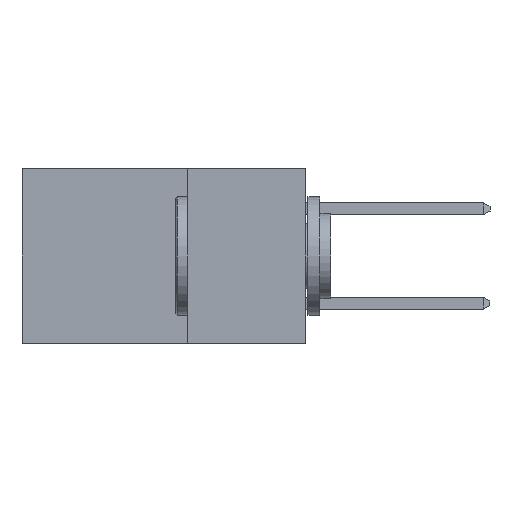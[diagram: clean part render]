
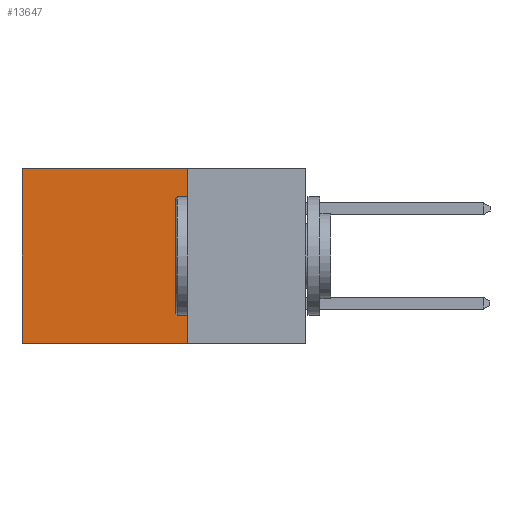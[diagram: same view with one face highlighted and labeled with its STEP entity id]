
A CAD part, left-side view. The second image highlights one B-rep face of the part: STEP entity #13647.
In plain terms, the highlighted planar face has unit normal (-1, 0, 0).
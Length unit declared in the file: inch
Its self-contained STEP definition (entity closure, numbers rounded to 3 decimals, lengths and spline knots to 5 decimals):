
#135 = EDGE_LOOP ( 'NONE', ( #23968, #1045, #19293, #12222 ) ) ;
#969 = CARTESIAN_POINT ( 'NONE',  ( 0.298, 0.25, -0.37 ) ) ;
#1045 = ORIENTED_EDGE ( 'NONE', *, *, #22893, .F. ) ;
#1444 = LINE ( 'NONE', #969, #5917 ) ;
#2767 = CARTESIAN_POINT ( 'NONE',  ( 0.298, 0.25, 0. ) ) ;
#2989 = CARTESIAN_POINT ( 'NONE',  ( 0.298, 0.25, 0. ) ) ;
#3025 = CARTESIAN_POINT ( 'NONE',  ( 0.298, 0.6, -0.37 ) ) ;
#3817 = EDGE_CURVE ( 'NONE', #9918, #7868, #16324, .T. ) ;
#3919 = VERTEX_POINT ( 'NONE', #2767 ) ;
#4996 = CARTESIAN_POINT ( 'NONE',  ( 0.298, 0.25, 0. ) ) ;
#5917 = VECTOR ( 'NONE', #16052, 39.37008 ) ;
#5967 = FACE_OUTER_BOUND ( 'NONE', #135, .T. ) ;
#6118 = AXIS2_PLACEMENT_3D ( 'NONE', #2989, #8831, #21843 ) ;
#6264 = CARTESIAN_POINT ( 'NONE',  ( 0.298, 0.6, 0. ) ) ;
#6275 = DIRECTION ( 'NONE',  ( 0., 0., -1. ) ) ;
#6804 = LINE ( 'NONE', #15313, #15561 ) ;
#6975 = VECTOR ( 'NONE', #6275, 39.37008 ) ;
#7868 = VERTEX_POINT ( 'NONE', #3025 ) ;
#8831 = DIRECTION ( 'NONE',  ( 1., 0., 0. ) ) ;
#9918 = VERTEX_POINT ( 'NONE', #20665 ) ;
#10647 = PLANE ( 'NONE',  #6118 ) ;
#11570 = DIRECTION ( 'NONE',  ( 0., 0., -1. ) ) ;
#12222 = ORIENTED_EDGE ( 'NONE', *, *, #14434, .T. ) ;
#13647 = ADVANCED_FACE ( 'NONE', ( #5967 ), #10647, .F. ) ;
#13958 = VECTOR ( 'NONE', #20017, 39.37008 ) ;
#14434 = EDGE_CURVE ( 'NONE', #3919, #9918, #19519, .T. ) ;
#14982 = VERTEX_POINT ( 'NONE', #17824 ) ;
#15313 = CARTESIAN_POINT ( 'NONE',  ( 0.298, 0.25, 0. ) ) ;
#15561 = VECTOR ( 'NONE', #11570, 39.37008 ) ;
#16052 = DIRECTION ( 'NONE',  ( 0., 1., 0. ) ) ;
#16324 = LINE ( 'NONE', #6264, #6975 ) ;
#17824 = CARTESIAN_POINT ( 'NONE',  ( 0.298, 0.25, -0.37 ) ) ;
#19293 = ORIENTED_EDGE ( 'NONE', *, *, #23530, .F. ) ;
#19519 = LINE ( 'NONE', #4996, #13958 ) ;
#20017 = DIRECTION ( 'NONE',  ( 0., 1., 0. ) ) ;
#20665 = CARTESIAN_POINT ( 'NONE',  ( 0.298, 0.6, 0. ) ) ;
#21843 = DIRECTION ( 'NONE',  ( 0., 0., -1. ) ) ;
#22893 = EDGE_CURVE ( 'NONE', #14982, #7868, #1444, .T. ) ;
#23530 = EDGE_CURVE ( 'NONE', #3919, #14982, #6804, .T. ) ;
#23968 = ORIENTED_EDGE ( 'NONE', *, *, #3817, .T. ) ;
